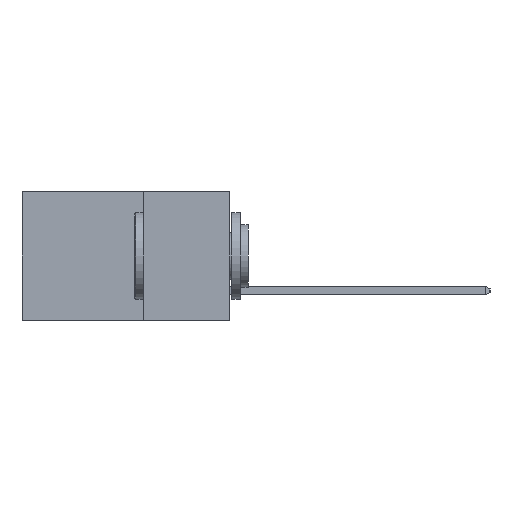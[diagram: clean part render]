
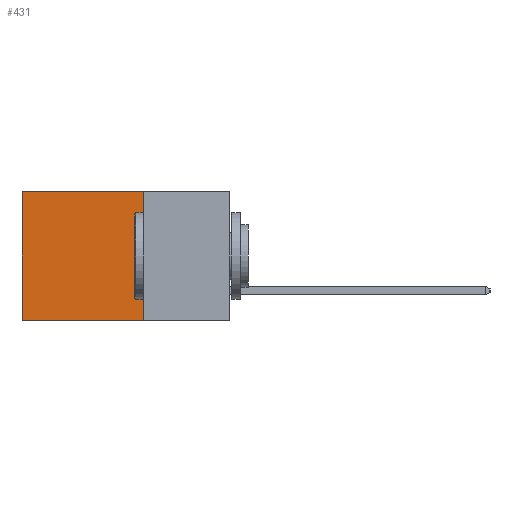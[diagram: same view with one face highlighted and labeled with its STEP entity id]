
A CAD part, left-side view. The second image highlights one B-rep face of the part: STEP entity #431.
In plain terms, the highlighted planar face has unit normal (-1, 0, 0).
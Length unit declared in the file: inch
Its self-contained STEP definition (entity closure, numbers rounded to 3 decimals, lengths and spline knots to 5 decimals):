
#369 = ORIENTED_EDGE ( 'NONE', *, *, #9956, .F. ) ;
#431 = ADVANCED_FACE ( 'NONE', ( #6859 ), #4063, .F. ) ;
#605 = ORIENTED_EDGE ( 'NONE', *, *, #9991, .F. ) ;
#883 = DIRECTION ( 'NONE',  ( 1., 0., 0. ) ) ;
#1617 = LINE ( 'NONE', #9360, #2026 ) ;
#1640 = EDGE_LOOP ( 'NONE', ( #3282, #369, #605, #4874 ) ) ;
#1787 = CARTESIAN_POINT ( 'NONE',  ( 0.298, 0.25, -0.37 ) ) ;
#2026 = VECTOR ( 'NONE', #11264, 39.37008 ) ;
#2841 = AXIS2_PLACEMENT_3D ( 'NONE', #5764, #883, #3907 ) ;
#3282 = ORIENTED_EDGE ( 'NONE', *, *, #4760, .T. ) ;
#3907 = DIRECTION ( 'NONE',  ( 0., 0., -1. ) ) ;
#4063 = PLANE ( 'NONE',  #2841 ) ;
#4379 = VERTEX_POINT ( 'NONE', #13395 ) ;
#4760 = EDGE_CURVE ( 'NONE', #9230, #5095, #1617, .T. ) ;
#4874 = ORIENTED_EDGE ( 'NONE', *, *, #7438, .T. ) ;
#5095 = VERTEX_POINT ( 'NONE', #9665 ) ;
#5267 = LINE ( 'NONE', #8386, #11290 ) ;
#5286 = VERTEX_POINT ( 'NONE', #11145 ) ;
#5713 = DIRECTION ( 'NONE',  ( 0., 1., 0. ) ) ;
#5764 = CARTESIAN_POINT ( 'NONE',  ( 0.298, 0.25, 0. ) ) ;
#5972 = LINE ( 'NONE', #9863, #12369 ) ;
#6396 = LINE ( 'NONE', #1787, #16346 ) ;
#6859 = FACE_OUTER_BOUND ( 'NONE', #1640, .T. ) ;
#7438 = EDGE_CURVE ( 'NONE', #4379, #9230, #5267, .T. ) ;
#8386 = CARTESIAN_POINT ( 'NONE',  ( 0.298, 0.25, 0. ) ) ;
#9230 = VERTEX_POINT ( 'NONE', #12887 ) ;
#9360 = CARTESIAN_POINT ( 'NONE',  ( 0.298, 0.6, 0. ) ) ;
#9665 = CARTESIAN_POINT ( 'NONE',  ( 0.298, 0.6, -0.37 ) ) ;
#9863 = CARTESIAN_POINT ( 'NONE',  ( 0.298, 0.25, 0. ) ) ;
#9956 = EDGE_CURVE ( 'NONE', #5286, #5095, #6396, .T. ) ;
#9991 = EDGE_CURVE ( 'NONE', #4379, #5286, #5972, .T. ) ;
#10895 = DIRECTION ( 'NONE',  ( 0., 1., 0. ) ) ;
#11106 = DIRECTION ( 'NONE',  ( 0., 0., -1. ) ) ;
#11145 = CARTESIAN_POINT ( 'NONE',  ( 0.298, 0.25, -0.37 ) ) ;
#11264 = DIRECTION ( 'NONE',  ( 0., 0., -1. ) ) ;
#11290 = VECTOR ( 'NONE', #5713, 39.37008 ) ;
#12369 = VECTOR ( 'NONE', #11106, 39.37008 ) ;
#12887 = CARTESIAN_POINT ( 'NONE',  ( 0.298, 0.6, 0. ) ) ;
#13395 = CARTESIAN_POINT ( 'NONE',  ( 0.298, 0.25, 0. ) ) ;
#16346 = VECTOR ( 'NONE', #10895, 39.37008 ) ;
